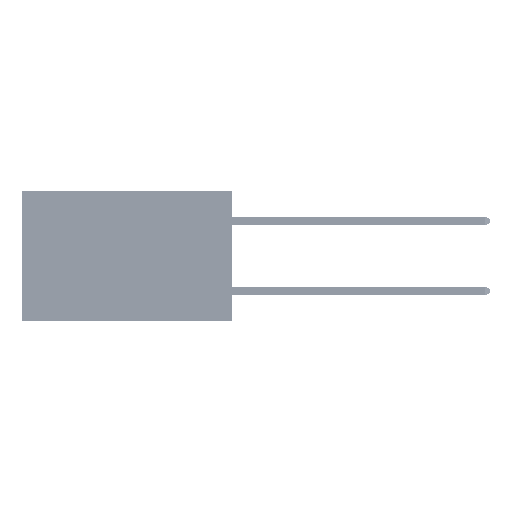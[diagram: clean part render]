
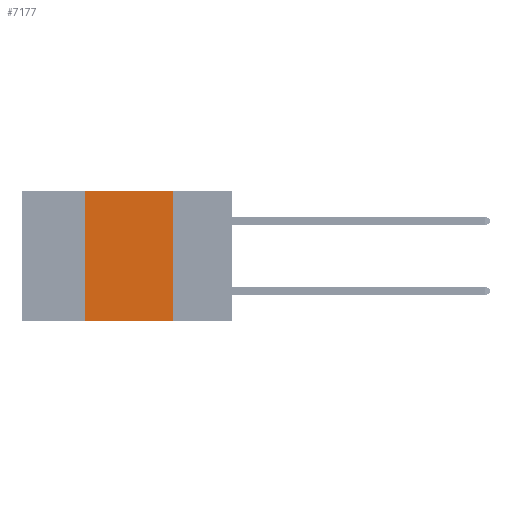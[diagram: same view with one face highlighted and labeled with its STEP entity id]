
A CAD part, left-side view. The second image highlights one B-rep face of the part: STEP entity #7177.
In plain terms, the highlighted planar face has unit normal (-1, 0, 0).
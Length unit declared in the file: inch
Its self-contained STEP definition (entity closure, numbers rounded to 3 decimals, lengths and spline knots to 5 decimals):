
#683 = EDGE_CURVE ( 'NONE', #39890, #38156, #38539, .T. ) ;
#2866 = CARTESIAN_POINT ( 'NONE',  ( 0., 0.42, 0. ) ) ;
#6247 = ORIENTED_EDGE ( 'NONE', *, *, #6637, .T. ) ;
#6386 = LINE ( 'NONE', #38959, #33063 ) ;
#6637 = EDGE_CURVE ( 'NONE', #39890, #25071, #42615, .T. ) ;
#7106 = FACE_OUTER_BOUND ( 'NONE', #49386, .T. ) ;
#7177 = ADVANCED_FACE ( 'NONE', ( #7106 ), #33888, .F. ) ;
#8090 = VECTOR ( 'NONE', #22974, 39.37008 ) ;
#8105 = VERTEX_POINT ( 'NONE', #32600 ) ;
#14664 = VECTOR ( 'NONE', #19076, 39.37008 ) ;
#19076 = DIRECTION ( 'NONE',  ( 0., -1., 0. ) ) ;
#22157 = LINE ( 'NONE', #26763, #14664 ) ;
#22974 = DIRECTION ( 'NONE',  ( 0., 0., 1. ) ) ;
#25071 = VERTEX_POINT ( 'NONE', #28136 ) ;
#25956 = CARTESIAN_POINT ( 'NONE',  ( 0., 0.6, 0. ) ) ;
#26361 = CARTESIAN_POINT ( 'NONE',  ( 0., 0.6, -0.37 ) ) ;
#26667 = ORIENTED_EDGE ( 'NONE', *, *, #28867, .F. ) ;
#26763 = CARTESIAN_POINT ( 'NONE',  ( 0., 0.6, 0. ) ) ;
#28136 = CARTESIAN_POINT ( 'NONE',  ( 0., 0.17, -0.37 ) ) ;
#28867 = EDGE_CURVE ( 'NONE', #38156, #8105, #22157, .T. ) ;
#30045 = AXIS2_PLACEMENT_3D ( 'NONE', #25956, #45357, #45868 ) ;
#30850 = CARTESIAN_POINT ( 'NONE',  ( 0., 0.42, -0.37 ) ) ;
#32113 = CARTESIAN_POINT ( 'NONE',  ( 0., 0.42, 0. ) ) ;
#32600 = CARTESIAN_POINT ( 'NONE',  ( 0., 0.17, 0. ) ) ;
#33063 = VECTOR ( 'NONE', #39141, 39.37008 ) ;
#33888 = PLANE ( 'NONE',  #30045 ) ;
#34481 = DIRECTION ( 'NONE',  ( 0., -1., 0. ) ) ;
#37155 = EDGE_CURVE ( 'NONE', #8105, #25071, #6386, .T. ) ;
#38156 = VERTEX_POINT ( 'NONE', #32113 ) ;
#38539 = LINE ( 'NONE', #2866, #8090 ) ;
#38959 = CARTESIAN_POINT ( 'NONE',  ( 0., 0.17, 0. ) ) ;
#39141 = DIRECTION ( 'NONE',  ( 0., 0., -1. ) ) ;
#39890 = VERTEX_POINT ( 'NONE', #30850 ) ;
#40575 = ORIENTED_EDGE ( 'NONE', *, *, #37155, .F. ) ;
#42615 = LINE ( 'NONE', #26361, #48144 ) ;
#43615 = ORIENTED_EDGE ( 'NONE', *, *, #683, .F. ) ;
#45357 = DIRECTION ( 'NONE',  ( 1., 0., 0. ) ) ;
#45868 = DIRECTION ( 'NONE',  ( 0., 0., -1. ) ) ;
#48144 = VECTOR ( 'NONE', #34481, 39.37008 ) ;
#49386 = EDGE_LOOP ( 'NONE', ( #40575, #26667, #43615, #6247 ) ) ;
